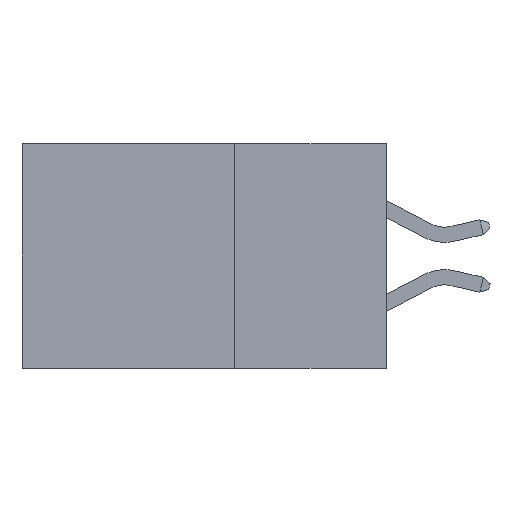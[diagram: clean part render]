
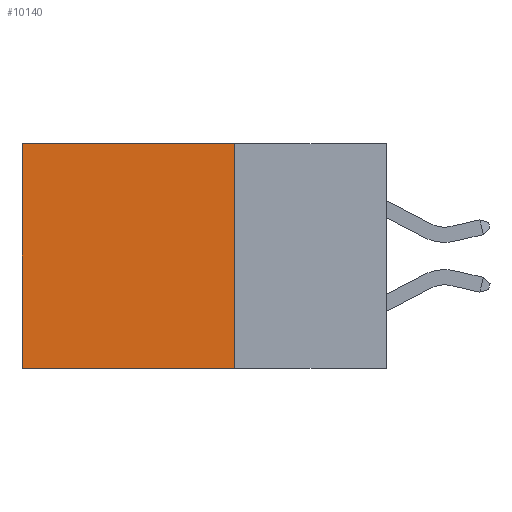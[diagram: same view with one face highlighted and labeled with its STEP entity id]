
A CAD part, left-side view. The second image highlights one B-rep face of the part: STEP entity #10140.
In plain terms, the highlighted planar face has unit normal (-1, 0, 0).
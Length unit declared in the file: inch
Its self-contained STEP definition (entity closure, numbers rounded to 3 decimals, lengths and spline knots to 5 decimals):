
#368 = VECTOR ( 'NONE', #7741, 39.37008 ) ;
#408 = DIRECTION ( 'NONE',  ( 0., 0., -1. ) ) ;
#435 = EDGE_CURVE ( 'NONE', #8349, #5812, #4860, .T. ) ;
#2298 = VERTEX_POINT ( 'NONE', #5608 ) ;
#2583 = CARTESIAN_POINT ( 'NONE',  ( 0.298, 0.25, 0. ) ) ;
#3030 = ORIENTED_EDGE ( 'NONE', *, *, #9699, .T. ) ;
#3451 = CARTESIAN_POINT ( 'NONE',  ( 0.298, 0.25, -0.37 ) ) ;
#3569 = PLANE ( 'NONE',  #4113 ) ;
#3634 = ORIENTED_EDGE ( 'NONE', *, *, #3818, .F. ) ;
#3818 = EDGE_CURVE ( 'NONE', #2298, #5328, #4385, .T. ) ;
#3836 = LINE ( 'NONE', #10627, #5261 ) ;
#4026 = FACE_OUTER_BOUND ( 'NONE', #9191, .T. ) ;
#4113 = AXIS2_PLACEMENT_3D ( 'NONE', #8540, #7816, #408 ) ;
#4385 = LINE ( 'NONE', #6132, #368 ) ;
#4681 = CARTESIAN_POINT ( 'NONE',  ( 0.298, 0.6, -0.37 ) ) ;
#4691 = VECTOR ( 'NONE', #8287, 39.37008 ) ;
#4860 = LINE ( 'NONE', #6496, #7336 ) ;
#5261 = VECTOR ( 'NONE', #5672, 39.37008 ) ;
#5328 = VERTEX_POINT ( 'NONE', #3451 ) ;
#5386 = CARTESIAN_POINT ( 'NONE',  ( 0.298, 0.6, 0. ) ) ;
#5608 = CARTESIAN_POINT ( 'NONE',  ( 0.298, 0.25, 0. ) ) ;
#5672 = DIRECTION ( 'NONE',  ( 0., 1., 0. ) ) ;
#5711 = DIRECTION ( 'NONE',  ( 0., 0., -1. ) ) ;
#5812 = VERTEX_POINT ( 'NONE', #4681 ) ;
#6132 = CARTESIAN_POINT ( 'NONE',  ( 0.298, 0.25, 0. ) ) ;
#6219 = EDGE_CURVE ( 'NONE', #5328, #5812, #3836, .T. ) ;
#6496 = CARTESIAN_POINT ( 'NONE',  ( 0.298, 0.6, 0. ) ) ;
#6891 = LINE ( 'NONE', #2583, #4691 ) ;
#7336 = VECTOR ( 'NONE', #5711, 39.37008 ) ;
#7533 = ORIENTED_EDGE ( 'NONE', *, *, #435, .T. ) ;
#7741 = DIRECTION ( 'NONE',  ( 0., 0., -1. ) ) ;
#7816 = DIRECTION ( 'NONE',  ( 1., 0., 0. ) ) ;
#8287 = DIRECTION ( 'NONE',  ( 0., 1., 0. ) ) ;
#8349 = VERTEX_POINT ( 'NONE', #5386 ) ;
#8540 = CARTESIAN_POINT ( 'NONE',  ( 0.298, 0.25, 0. ) ) ;
#9191 = EDGE_LOOP ( 'NONE', ( #7533, #9760, #3634, #3030 ) ) ;
#9699 = EDGE_CURVE ( 'NONE', #2298, #8349, #6891, .T. ) ;
#9760 = ORIENTED_EDGE ( 'NONE', *, *, #6219, .F. ) ;
#10140 = ADVANCED_FACE ( 'NONE', ( #4026 ), #3569, .F. ) ;
#10627 = CARTESIAN_POINT ( 'NONE',  ( 0.298, 0.25, -0.37 ) ) ;
